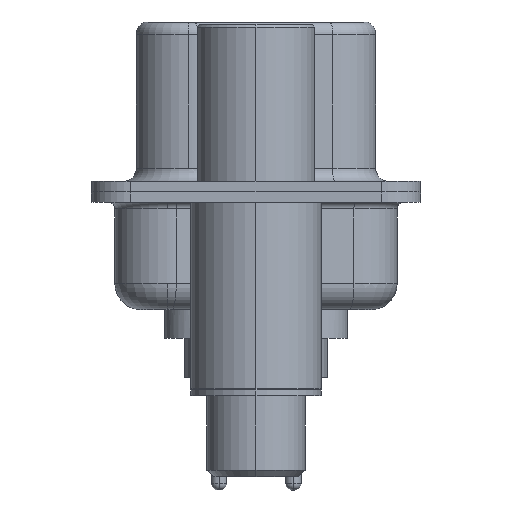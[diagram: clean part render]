
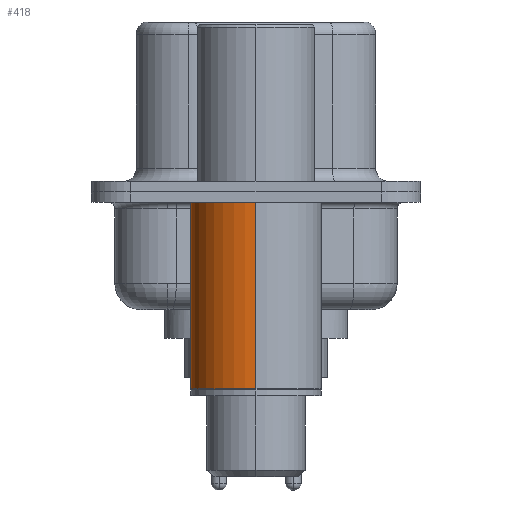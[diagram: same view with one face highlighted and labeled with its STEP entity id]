
A CAD part, left-side view. The second image highlights one B-rep face of the part: STEP entity #418.
In plain terms, the highlighted cylindrical face has radius 2.5 mm (diameter 5 mm), a partial arc.
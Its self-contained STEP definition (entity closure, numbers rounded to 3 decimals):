
#418 = ADVANCED_FACE ( 'NONE', ( #9310 ), #4510, .T. ) ;
#915 = CARTESIAN_POINT ( 'NONE',  ( 0., 0., -7.525 ) ) ;
#2359 = DIRECTION ( 'NONE',  ( 0., 0., 1. ) ) ;
#2647 = VERTEX_POINT ( 'NONE', #18957 ) ;
#3208 = CARTESIAN_POINT ( 'NONE',  ( 0., 0., 0.581 ) ) ;
#4008 = VECTOR ( 'NONE', #10360, 1000. ) ;
#4343 = ORIENTED_EDGE ( 'NONE', *, *, #21069, .T. ) ;
#4417 = DIRECTION ( 'NONE',  ( 1., 0., 0. ) ) ;
#4510 = CYLINDRICAL_SURFACE ( 'NONE', #20242, 2.5 ) ;
#4696 = EDGE_LOOP ( 'NONE', ( #4343, #11753, #18967, #26549 ) ) ;
#5696 = EDGE_CURVE ( 'NONE', #2647, #7956, #7225, .T. ) ;
#7225 = LINE ( 'NONE', #14530, #4008 ) ;
#7312 = CIRCLE ( 'NONE', #9661, 2.5 ) ;
#7956 = VERTEX_POINT ( 'NONE', #12280 ) ;
#8485 = CARTESIAN_POINT ( 'NONE',  ( 0., 0., -0.4 ) ) ;
#9310 = FACE_OUTER_BOUND ( 'NONE', #4696, .T. ) ;
#9333 = DIRECTION ( 'NONE',  ( 0., 0., 1. ) ) ;
#9509 = CIRCLE ( 'NONE', #15890, 2.5 ) ;
#9661 = AXIS2_PLACEMENT_3D ( 'NONE', #915, #17258, #4417 ) ;
#10256 = EDGE_CURVE ( 'NONE', #10889, #17521, #13372, .T. ) ;
#10360 = DIRECTION ( 'NONE',  ( 0., 0., 1. ) ) ;
#10889 = VERTEX_POINT ( 'NONE', #24847 ) ;
#11753 = ORIENTED_EDGE ( 'NONE', *, *, #5696, .T. ) ;
#12280 = CARTESIAN_POINT ( 'NONE',  ( -2.5, 0., -0.4 ) ) ;
#13372 = LINE ( 'NONE', #25412, #24848 ) ;
#13680 = CARTESIAN_POINT ( 'NONE',  ( 2.5, 0., -0.4 ) ) ;
#14530 = CARTESIAN_POINT ( 'NONE',  ( -2.5, 0., 0.581 ) ) ;
#15890 = AXIS2_PLACEMENT_3D ( 'NONE', #8485, #2359, #25355 ) ;
#17258 = DIRECTION ( 'NONE',  ( 0., 0., 1. ) ) ;
#17521 = VERTEX_POINT ( 'NONE', #13680 ) ;
#18957 = CARTESIAN_POINT ( 'NONE',  ( -2.5, 0., -7.525 ) ) ;
#18967 = ORIENTED_EDGE ( 'NONE', *, *, #22250, .F. ) ;
#19709 = DIRECTION ( 'NONE',  ( 1., 0., 0. ) ) ;
#20242 = AXIS2_PLACEMENT_3D ( 'NONE', #3208, #21663, #19709 ) ;
#21069 = EDGE_CURVE ( 'NONE', #10889, #2647, #7312, .T. ) ;
#21663 = DIRECTION ( 'NONE',  ( 0., 0., 1. ) ) ;
#22250 = EDGE_CURVE ( 'NONE', #17521, #7956, #9509, .T. ) ;
#24847 = CARTESIAN_POINT ( 'NONE',  ( 2.5, 0., -7.525 ) ) ;
#24848 = VECTOR ( 'NONE', #9333, 1000. ) ;
#25355 = DIRECTION ( 'NONE',  ( 1., 0., 0. ) ) ;
#25412 = CARTESIAN_POINT ( 'NONE',  ( 2.5, 0., 0.581 ) ) ;
#26549 = ORIENTED_EDGE ( 'NONE', *, *, #10256, .F. ) ;
